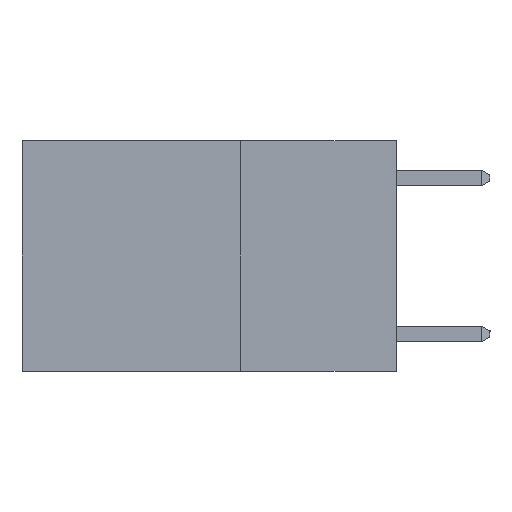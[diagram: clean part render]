
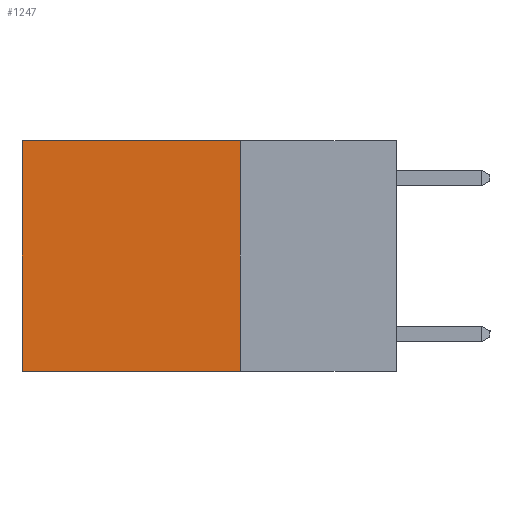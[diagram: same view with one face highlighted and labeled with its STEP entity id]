
A CAD part, left-side view. The second image highlights one B-rep face of the part: STEP entity #1247.
In plain terms, the highlighted planar face has unit normal (-1, 0, 0).
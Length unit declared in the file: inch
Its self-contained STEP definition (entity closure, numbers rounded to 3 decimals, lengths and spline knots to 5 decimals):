
#660 = CARTESIAN_POINT ( 'NONE',  ( 0.2625, 0.25, 0. ) ) ;
#692 = VECTOR ( 'NONE', #2360, 39.37008 ) ;
#853 = FACE_OUTER_BOUND ( 'NONE', #3359, .T. ) ;
#1144 = EDGE_CURVE ( 'NONE', #4606, #10441, #6864, .T. ) ;
#1247 = ADVANCED_FACE ( 'NONE', ( #853 ), #4324, .F. ) ;
#2360 = DIRECTION ( 'NONE',  ( 0., 1., 0. ) ) ;
#2568 = LINE ( 'NONE', #660, #10790 ) ;
#3165 = ORIENTED_EDGE ( 'NONE', *, *, #10449, .T. ) ;
#3266 = CARTESIAN_POINT ( 'NONE',  ( 0.2625, 0.25, 0. ) ) ;
#3359 = EDGE_LOOP ( 'NONE', ( #3165, #9628, #4973, #8054 ) ) ;
#3442 = DIRECTION ( 'NONE',  ( 0., 0., -1. ) ) ;
#3513 = DIRECTION ( 'NONE',  ( 0., 0., -1. ) ) ;
#3710 = AXIS2_PLACEMENT_3D ( 'NONE', #6823, #8472, #3513 ) ;
#3943 = DIRECTION ( 'NONE',  ( 0., 1., 0. ) ) ;
#3977 = DIRECTION ( 'NONE',  ( 0., 0., -1. ) ) ;
#4324 = PLANE ( 'NONE',  #3710 ) ;
#4606 = VERTEX_POINT ( 'NONE', #3266 ) ;
#4737 = CARTESIAN_POINT ( 'NONE',  ( 0.2625, 0.25, -0.37 ) ) ;
#4868 = CARTESIAN_POINT ( 'NONE',  ( 0.2625, 0.25, 0. ) ) ;
#4973 = ORIENTED_EDGE ( 'NONE', *, *, #8465, .F. ) ;
#5196 = VECTOR ( 'NONE', #3977, 39.37008 ) ;
#5755 = VECTOR ( 'NONE', #3943, 39.37008 ) ;
#6823 = CARTESIAN_POINT ( 'NONE',  ( 0.2625, 0.25, 0. ) ) ;
#6864 = LINE ( 'NONE', #4868, #692 ) ;
#7386 = LINE ( 'NONE', #10474, #5196 ) ;
#7864 = CARTESIAN_POINT ( 'NONE',  ( 0.2625, 0.6, -0.37 ) ) ;
#7946 = LINE ( 'NONE', #4737, #5755 ) ;
#8037 = EDGE_CURVE ( 'NONE', #10775, #10912, #7946, .T. ) ;
#8054 = ORIENTED_EDGE ( 'NONE', *, *, #1144, .T. ) ;
#8099 = CARTESIAN_POINT ( 'NONE',  ( 0.2625, 0.6, 0. ) ) ;
#8465 = EDGE_CURVE ( 'NONE', #4606, #10775, #2568, .T. ) ;
#8472 = DIRECTION ( 'NONE',  ( 1., 0., 0. ) ) ;
#9628 = ORIENTED_EDGE ( 'NONE', *, *, #8037, .F. ) ;
#10133 = CARTESIAN_POINT ( 'NONE',  ( 0.2625, 0.25, -0.37 ) ) ;
#10441 = VERTEX_POINT ( 'NONE', #8099 ) ;
#10449 = EDGE_CURVE ( 'NONE', #10441, #10912, #7386, .T. ) ;
#10474 = CARTESIAN_POINT ( 'NONE',  ( 0.2625, 0.6, 0. ) ) ;
#10775 = VERTEX_POINT ( 'NONE', #10133 ) ;
#10790 = VECTOR ( 'NONE', #3442, 39.37008 ) ;
#10912 = VERTEX_POINT ( 'NONE', #7864 ) ;
